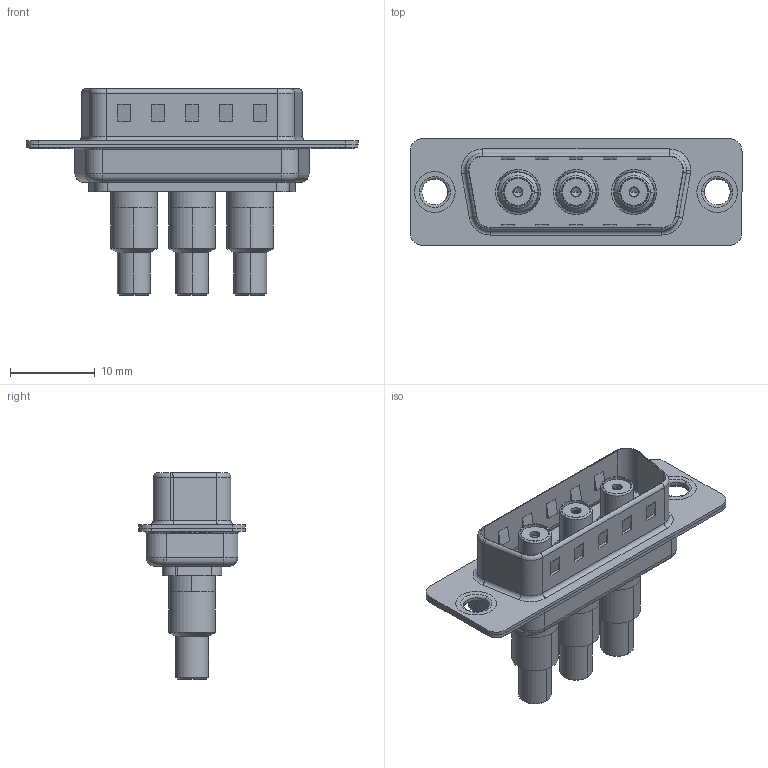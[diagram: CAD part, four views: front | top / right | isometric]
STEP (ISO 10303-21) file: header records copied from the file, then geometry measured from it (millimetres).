
FILE_DESCRIPTION (( 'STEP AP203' ), '1' );
FILE_NAME ('627-3W3-622-5T1.STEP', '2019-05-24T16:32:35', ( '' ), ( '' ), 'SwSTEP 2.0', 'SolidWorks 2016', '' );
FILE_SCHEMA (( 'CONFIG_CONTROL_DESIGN' ));
Length unit declared in the file: millimetre
Products named in the file (12): Insulator Socket; Insulator Socket 2; Locking Collar; Socket_Solder Cup; 627Combo Housing_3W3; Solder Cover; 627Combo Shell Rear_15 Contacts; Co-Ax Jack Assy_SC; 627Combo Shell Front_15 Contacts; 627-3W3-622-5T1; 627Combo Thru Hole Rivet; Co-Ax Jack_Solder Cup Tail
Assembly tree (14 placements, depth 3):
  627-3W3-622-5T1
    627Combo Housing_3W3
    627Combo Shell Rear_15 Contacts
    627Combo Shell Front_15 Contacts
    627Combo Thru Hole Rivet  x2
    Co-Ax Jack Assy_SC  x3
      Co-Ax Jack_Solder Cup Tail
      Insulator Socket
      Insulator Socket 2
      Locking Collar
      Socket_Solder Cup
      Solder Cover
Bounding box: 39.15 x 12.6 x 24.3 mm (x, y, z)
Volume: 2146.6 mm3; surface area: 7068.9 mm2
Topology: 23 solids, 23 shells, 704 faces, 1642 edges, 1010 vertices
Faces by surface type: cylinder 309, plane 259, torus 70, cone 60, bspline 6
Entity records: 14216 total; most frequent: DIRECTION 2364, CARTESIAN_POINT 2335, ORIENTED_EDGE 2084, EDGE_CURVE 1042, AXIS2_PLACEMENT_3D 901, VERTEX_POINT 650, VECTOR 562, LINE 562
